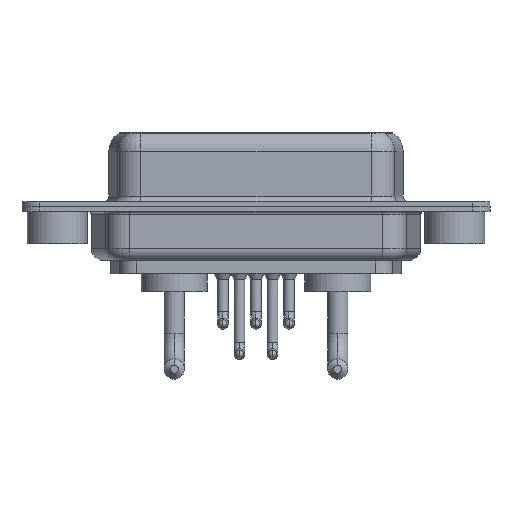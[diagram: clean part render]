
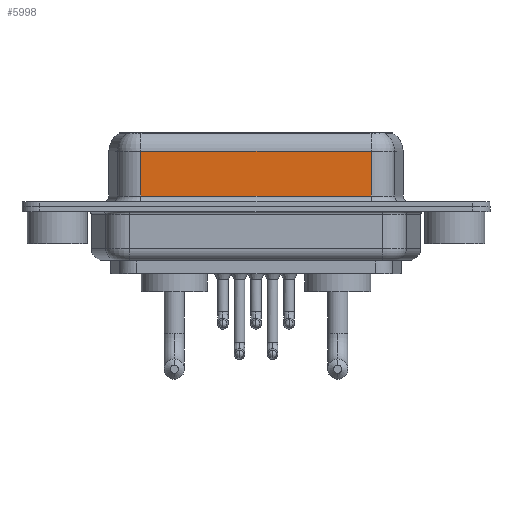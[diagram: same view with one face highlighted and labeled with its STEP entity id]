
A CAD part, front view. The second image highlights one B-rep face of the part: STEP entity #5998.
In plain terms, the highlighted planar face has unit normal (0, -1, 0).
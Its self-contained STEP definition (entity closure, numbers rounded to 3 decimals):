
#413 = FACE_OUTER_BOUND ( 'NONE', #13076, .T. ) ;
#521 = DIRECTION ( 'NONE',  ( 1., 0., 0. ) ) ;
#548 = EDGE_CURVE ( 'NONE', #11753, #15382, #764, .T. ) ;
#764 = LINE ( 'NONE', #14929, #10817 ) ;
#1793 = PLANE ( 'NONE',  #10110 ) ;
#2521 = ORIENTED_EDGE ( 'NONE', *, *, #15686, .F. ) ;
#3325 = LINE ( 'NONE', #6134, #16708 ) ;
#3333 = ORIENTED_EDGE ( 'NONE', *, *, #8753, .T. ) ;
#4145 = DIRECTION ( 'NONE',  ( 0., 0., -1. ) ) ;
#4467 = CARTESIAN_POINT ( 'NONE',  ( 26.287, -3.95, 0.9 ) ) ;
#4771 = DIRECTION ( 'NONE',  ( 0., 0., -1. ) ) ;
#5748 = LINE ( 'NONE', #4467, #8035 ) ;
#5998 = ADVANCED_FACE ( 'NONE', ( #413 ), #1793, .F. ) ;
#6059 = DIRECTION ( 'NONE',  ( -1., 0., 0. ) ) ;
#6134 = CARTESIAN_POINT ( 'NONE',  ( 7.013, -3.95, 6.4 ) ) ;
#6657 = VECTOR ( 'NONE', #4145, 1000. ) ;
#6996 = DIRECTION ( 'NONE',  ( 0., 0., 1. ) ) ;
#8035 = VECTOR ( 'NONE', #521, 1000. ) ;
#8446 = CARTESIAN_POINT ( 'NONE',  ( 26.287, -3.95, 6.4 ) ) ;
#8745 = VERTEX_POINT ( 'NONE', #9719 ) ;
#8753 = EDGE_CURVE ( 'NONE', #15382, #8745, #3325, .T. ) ;
#8778 = CARTESIAN_POINT ( 'NONE',  ( 26.287, -3.95, 0.9 ) ) ;
#9033 = VERTEX_POINT ( 'NONE', #8778 ) ;
#9188 = CARTESIAN_POINT ( 'NONE',  ( 26.287, -3.95, 6.4 ) ) ;
#9719 = CARTESIAN_POINT ( 'NONE',  ( 7.013, -3.95, 0.9 ) ) ;
#10087 = CARTESIAN_POINT ( 'NONE',  ( 7.013, -3.95, 4.65 ) ) ;
#10110 = AXIS2_PLACEMENT_3D ( 'NONE', #8446, #16029, #6996 ) ;
#10817 = VECTOR ( 'NONE', #6059, 1000. ) ;
#11753 = VERTEX_POINT ( 'NONE', #15064 ) ;
#13076 = EDGE_LOOP ( 'NONE', ( #2521, #15458, #3333, #15172 ) ) ;
#14371 = LINE ( 'NONE', #9188, #6657 ) ;
#14929 = CARTESIAN_POINT ( 'NONE',  ( 26.287, -3.95, 4.65 ) ) ;
#15064 = CARTESIAN_POINT ( 'NONE',  ( 26.287, -3.95, 4.65 ) ) ;
#15172 = ORIENTED_EDGE ( 'NONE', *, *, #16210, .T. ) ;
#15382 = VERTEX_POINT ( 'NONE', #10087 ) ;
#15458 = ORIENTED_EDGE ( 'NONE', *, *, #548, .T. ) ;
#15686 = EDGE_CURVE ( 'NONE', #11753, #9033, #14371, .T. ) ;
#16029 = DIRECTION ( 'NONE',  ( 0., 1., 0. ) ) ;
#16210 = EDGE_CURVE ( 'NONE', #8745, #9033, #5748, .T. ) ;
#16708 = VECTOR ( 'NONE', #4771, 1000. ) ;
